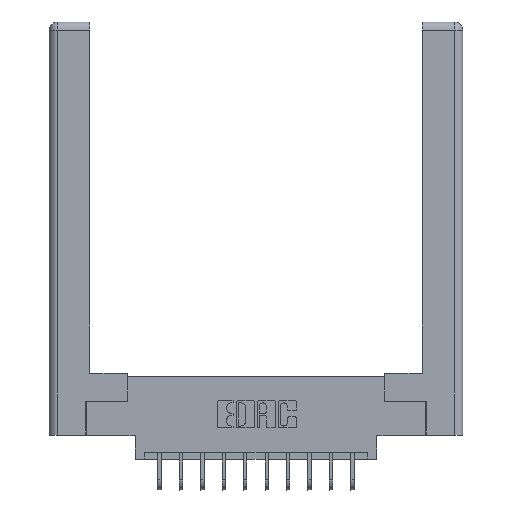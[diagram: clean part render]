
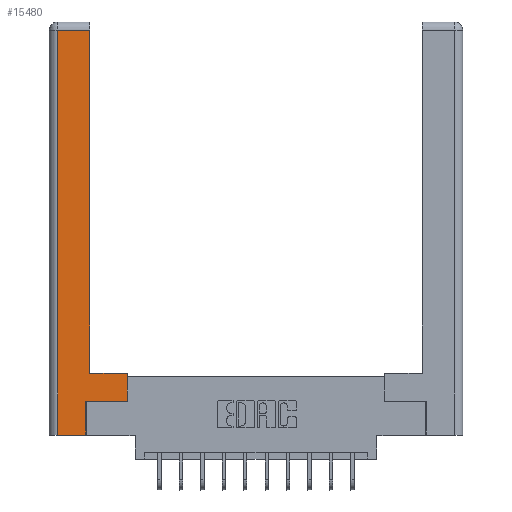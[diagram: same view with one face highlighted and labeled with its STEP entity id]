
A CAD part, top view. The second image highlights one B-rep face of the part: STEP entity #15480.
In plain terms, the highlighted planar face has unit normal (0, 0, 1).
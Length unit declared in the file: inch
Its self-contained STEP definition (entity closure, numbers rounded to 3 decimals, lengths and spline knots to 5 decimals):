
#184 = VERTEX_POINT ( 'NONE', #4065 ) ;
#255 = CARTESIAN_POINT ( 'NONE',  ( 0.265, 0., 0. ) ) ;
#285 = VECTOR ( 'NONE', #13028, 39.37008 ) ;
#304 = CARTESIAN_POINT ( 'NONE',  ( 0.265, 0.245, 0. ) ) ;
#366 = VERTEX_POINT ( 'NONE', #4391 ) ;
#503 = VECTOR ( 'NONE', #4154, 39.37008 ) ;
#584 = LINE ( 'NONE', #2199, #9535 ) ;
#617 = CARTESIAN_POINT ( 'NONE',  ( 0., 0., 0. ) ) ;
#727 = LINE ( 'NONE', #304, #10890 ) ;
#1759 = CARTESIAN_POINT ( 'NONE',  ( 0.295, 2.94, 0. ) ) ;
#2199 = CARTESIAN_POINT ( 'NONE',  ( 0.0615, 0., 0. ) ) ;
#2421 = VECTOR ( 'NONE', #9744, 39.37008 ) ;
#3269 = ORIENTED_EDGE ( 'NONE', *, *, #6643, .T. ) ;
#3823 = VECTOR ( 'NONE', #4290, 39.37008 ) ;
#3971 = EDGE_CURVE ( 'NONE', #10751, #14825, #7786, .T. ) ;
#4065 = CARTESIAN_POINT ( 'NONE',  ( 0.0615, 2.94, 0. ) ) ;
#4154 = DIRECTION ( 'NONE',  ( 0., 1., 0. ) ) ;
#4290 = DIRECTION ( 'NONE',  ( 1., 0., 0. ) ) ;
#4391 = CARTESIAN_POINT ( 'NONE',  ( 0.295, 0.45, 0. ) ) ;
#4429 = DIRECTION ( 'NONE',  ( 1., 0., 0. ) ) ;
#4472 = ORIENTED_EDGE ( 'NONE', *, *, #5120, .T. ) ;
#4745 = DIRECTION ( 'NONE',  ( -1., 0., 0. ) ) ;
#4950 = VERTEX_POINT ( 'NONE', #1759 ) ;
#4964 = FACE_OUTER_BOUND ( 'NONE', #7722, .T. ) ;
#5120 = EDGE_CURVE ( 'NONE', #184, #11819, #584, .T. ) ;
#5590 = LINE ( 'NONE', #16160, #5983 ) ;
#5641 = EDGE_CURVE ( 'NONE', #11819, #6712, #11705, .T. ) ;
#5983 = VECTOR ( 'NONE', #4745, 39.37008 ) ;
#6360 = CARTESIAN_POINT ( 'NONE',  ( 0.0615, 0., 0. ) ) ;
#6472 = ORIENTED_EDGE ( 'NONE', *, *, #3971, .T. ) ;
#6643 = EDGE_CURVE ( 'NONE', #6712, #10751, #727, .T. ) ;
#6712 = VERTEX_POINT ( 'NONE', #255 ) ;
#6927 = CARTESIAN_POINT ( 'NONE',  ( 0.565, 0.245, 0. ) ) ;
#7248 = CARTESIAN_POINT ( 'NONE',  ( 0.565, 0.45, 0. ) ) ;
#7338 = EDGE_CURVE ( 'NONE', #366, #4950, #14013, .T. ) ;
#7722 = EDGE_LOOP ( 'NONE', ( #10250, #10580, #4472, #15714, #3269, #6472, #14196, #10528 ) ) ;
#7786 = LINE ( 'NONE', #15490, #3823 ) ;
#7933 = VECTOR ( 'NONE', #4429, 39.37008 ) ;
#8119 = AXIS2_PLACEMENT_3D ( 'NONE', #617, #10749, #15787 ) ;
#9140 = CARTESIAN_POINT ( 'NONE',  ( 0.565, 0.45, 0. ) ) ;
#9535 = VECTOR ( 'NONE', #14887, 39.37008 ) ;
#9611 = CARTESIAN_POINT ( 'NONE',  ( 0.265, 0.245, 0. ) ) ;
#9744 = DIRECTION ( 'NONE',  ( 0., 1., 0. ) ) ;
#10250 = ORIENTED_EDGE ( 'NONE', *, *, #7338, .T. ) ;
#10478 = CARTESIAN_POINT ( 'NONE',  ( 0.295, 3., 0. ) ) ;
#10528 = ORIENTED_EDGE ( 'NONE', *, *, #14558, .T. ) ;
#10580 = ORIENTED_EDGE ( 'NONE', *, *, #11696, .T. ) ;
#10749 = DIRECTION ( 'NONE',  ( 0., 0., -1. ) ) ;
#10751 = VERTEX_POINT ( 'NONE', #9611 ) ;
#10756 = CARTESIAN_POINT ( 'NONE',  ( 0.265, 0., 0. ) ) ;
#10890 = VECTOR ( 'NONE', #14134, 39.37008 ) ;
#10996 = EDGE_CURVE ( 'NONE', #14825, #15408, #12553, .T. ) ;
#11696 = EDGE_CURVE ( 'NONE', #4950, #184, #5590, .T. ) ;
#11705 = LINE ( 'NONE', #10756, #7933 ) ;
#11819 = VERTEX_POINT ( 'NONE', #6360 ) ;
#11897 = PLANE ( 'NONE',  #8119 ) ;
#12553 = LINE ( 'NONE', #7248, #2421 ) ;
#13028 = DIRECTION ( 'NONE',  ( -1., 0., 0. ) ) ;
#14013 = LINE ( 'NONE', #10478, #503 ) ;
#14134 = DIRECTION ( 'NONE',  ( 0., 1., 0. ) ) ;
#14196 = ORIENTED_EDGE ( 'NONE', *, *, #10996, .T. ) ;
#14371 = LINE ( 'NONE', #15360, #285 ) ;
#14558 = EDGE_CURVE ( 'NONE', #15408, #366, #14371, .T. ) ;
#14825 = VERTEX_POINT ( 'NONE', #6927 ) ;
#14887 = DIRECTION ( 'NONE',  ( 0., -1., 0. ) ) ;
#15360 = CARTESIAN_POINT ( 'NONE',  ( 0.295, 0.45, 0. ) ) ;
#15408 = VERTEX_POINT ( 'NONE', #9140 ) ;
#15480 = ADVANCED_FACE ( 'NONE', ( #4964 ), #11897, .F. ) ;
#15490 = CARTESIAN_POINT ( 'NONE',  ( 0.565, 0.245, 0. ) ) ;
#15714 = ORIENTED_EDGE ( 'NONE', *, *, #5641, .T. ) ;
#15787 = DIRECTION ( 'NONE',  ( -1., 0., 0. ) ) ;
#16160 = CARTESIAN_POINT ( 'NONE',  ( 0.0615, 2.94, 0. ) ) ;
